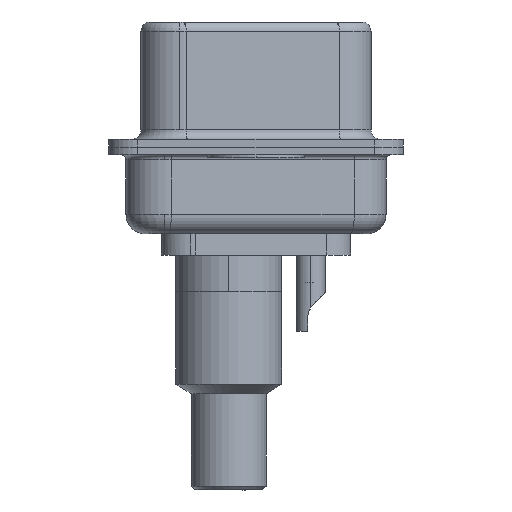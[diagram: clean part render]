
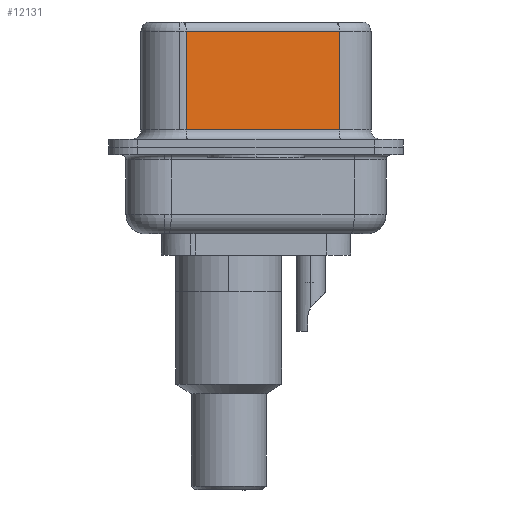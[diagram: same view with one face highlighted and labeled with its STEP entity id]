
A CAD part, left-side view. The second image highlights one B-rep face of the part: STEP entity #12131.
In plain terms, the highlighted planar face has unit normal (-0.985, -0.174, 0).
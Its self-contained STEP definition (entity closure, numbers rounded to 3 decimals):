
#54 = ORIENTED_EDGE ( 'NONE', *, *, #19319, .T. ) ;
#710 = LINE ( 'NONE', #14940, #22370 ) ;
#873 = VERTEX_POINT ( 'NONE', #14796 ) ;
#1751 = LINE ( 'NONE', #4296, #7587 ) ;
#2272 = VERTEX_POINT ( 'NONE', #24544 ) ;
#3159 = VERTEX_POINT ( 'NONE', #26935 ) ;
#4291 = EDGE_LOOP ( 'NONE', ( #10192, #5881, #12513, #54 ) ) ;
#4296 = CARTESIAN_POINT ( 'NONE',  ( 3.73, 3.628, 6.52 ) ) ;
#5703 = EDGE_CURVE ( 'NONE', #3159, #14611, #22991, .T. ) ;
#5881 = ORIENTED_EDGE ( 'NONE', *, *, #18479, .T. ) ;
#6494 = DIRECTION ( 'NONE',  ( 0., 0., -1. ) ) ;
#6753 = CARTESIAN_POINT ( 'NONE',  ( 5.132, -4.322, 6.52 ) ) ;
#7587 = VECTOR ( 'NONE', #6494, 1000. ) ;
#9260 = DIRECTION ( 'NONE',  ( 0.985, 0.174, 0. ) ) ;
#10192 = ORIENTED_EDGE ( 'NONE', *, *, #5703, .F. ) ;
#12016 = AXIS2_PLACEMENT_3D ( 'NONE', #22052, #9260, #24222 ) ;
#12131 = ADVANCED_FACE ( 'NONE', ( #14446 ), #19910, .F. ) ;
#12513 = ORIENTED_EDGE ( 'NONE', *, *, #18132, .T. ) ;
#14446 = FACE_OUTER_BOUND ( 'NONE', #4291, .T. ) ;
#14611 = VERTEX_POINT ( 'NONE', #23643 ) ;
#14796 = CARTESIAN_POINT ( 'NONE',  ( 3.73, 3.628, 0.9 ) ) ;
#14940 = CARTESIAN_POINT ( 'NONE',  ( 5.132, -4.322, 6.02 ) ) ;
#15652 = DIRECTION ( 'NONE',  ( 0.174, -0.985, 0. ) ) ;
#16057 = VECTOR ( 'NONE', #23181, 1000. ) ;
#18132 = EDGE_CURVE ( 'NONE', #2272, #873, #1751, .T. ) ;
#18479 = EDGE_CURVE ( 'NONE', #3159, #2272, #710, .T. ) ;
#19319 = EDGE_CURVE ( 'NONE', #873, #14611, #22009, .T. ) ;
#19910 = PLANE ( 'NONE',  #12016 ) ;
#22009 = LINE ( 'NONE', #26207, #22641 ) ;
#22052 = CARTESIAN_POINT ( 'NONE',  ( 5.132, -4.322, 6.52 ) ) ;
#22370 = VECTOR ( 'NONE', #23444, 1000. ) ;
#22641 = VECTOR ( 'NONE', #15652, 1000. ) ;
#22991 = LINE ( 'NONE', #6753, #16057 ) ;
#23181 = DIRECTION ( 'NONE',  ( 0., 0., -1. ) ) ;
#23444 = DIRECTION ( 'NONE',  ( -0.174, 0.985, 0. ) ) ;
#23643 = CARTESIAN_POINT ( 'NONE',  ( 5.132, -4.322, 0.9 ) ) ;
#24222 = DIRECTION ( 'NONE',  ( -0.174, 0.985, 0. ) ) ;
#24544 = CARTESIAN_POINT ( 'NONE',  ( 3.73, 3.628, 6.02 ) ) ;
#26207 = CARTESIAN_POINT ( 'NONE',  ( 5.132, -4.322, 0.9 ) ) ;
#26935 = CARTESIAN_POINT ( 'NONE',  ( 5.132, -4.322, 6.02 ) ) ;
